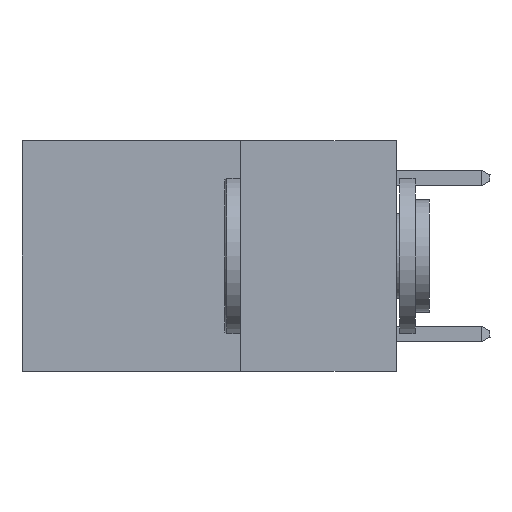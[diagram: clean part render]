
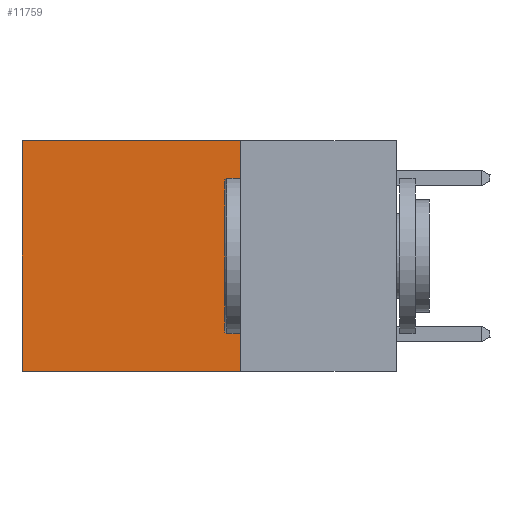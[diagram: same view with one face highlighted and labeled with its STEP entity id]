
A CAD part, left-side view. The second image highlights one B-rep face of the part: STEP entity #11759.
In plain terms, the highlighted planar face has unit normal (-1, 0, 0).
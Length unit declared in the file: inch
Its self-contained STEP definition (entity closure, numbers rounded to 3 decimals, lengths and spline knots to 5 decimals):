
#59 = DIRECTION ( 'NONE',  ( 0., 0., -1. ) ) ;
#110 = EDGE_CURVE ( 'NONE', #19671, #14846, #11611, .T. ) ;
#421 = DIRECTION ( 'NONE',  ( 0., 1., 0. ) ) ;
#1924 = DIRECTION ( 'NONE',  ( 0., 1., 0. ) ) ;
#2343 = CARTESIAN_POINT ( 'NONE',  ( 0.2625, 0.6, -0.37 ) ) ;
#3020 = CARTESIAN_POINT ( 'NONE',  ( 0.2625, 0.6, 0. ) ) ;
#3263 = LINE ( 'NONE', #19244, #4541 ) ;
#4438 = CARTESIAN_POINT ( 'NONE',  ( 0.2625, 0.25, 0. ) ) ;
#4541 = VECTOR ( 'NONE', #6297, 39.37008 ) ;
#6297 = DIRECTION ( 'NONE',  ( 0., 0., -1. ) ) ;
#6333 = CARTESIAN_POINT ( 'NONE',  ( 0.2625, 0.25, 0. ) ) ;
#6840 = VERTEX_POINT ( 'NONE', #6333 ) ;
#8144 = ORIENTED_EDGE ( 'NONE', *, *, #8543, .F. ) ;
#8543 = EDGE_CURVE ( 'NONE', #6840, #19671, #18642, .T. ) ;
#8999 = VECTOR ( 'NONE', #1924, 39.37008 ) ;
#9150 = AXIS2_PLACEMENT_3D ( 'NONE', #4438, #9249, #59 ) ;
#9249 = DIRECTION ( 'NONE',  ( 1., 0., 0. ) ) ;
#9448 = VERTEX_POINT ( 'NONE', #3020 ) ;
#9560 = PLANE ( 'NONE',  #9150 ) ;
#9979 = CARTESIAN_POINT ( 'NONE',  ( 0.2625, 0.25, 0. ) ) ;
#10255 = ORIENTED_EDGE ( 'NONE', *, *, #17837, .T. ) ;
#10469 = VECTOR ( 'NONE', #421, 39.37008 ) ;
#10628 = DIRECTION ( 'NONE',  ( 0., 0., -1. ) ) ;
#10818 = CARTESIAN_POINT ( 'NONE',  ( 0.2625, 0.25, 0. ) ) ;
#11611 = LINE ( 'NONE', #16772, #10469 ) ;
#11759 = ADVANCED_FACE ( 'NONE', ( #15549 ), #9560, .F. ) ;
#12289 = EDGE_LOOP ( 'NONE', ( #10255, #19639, #8144, #14338 ) ) ;
#13014 = LINE ( 'NONE', #9979, #8999 ) ;
#14338 = ORIENTED_EDGE ( 'NONE', *, *, #14637, .T. ) ;
#14637 = EDGE_CURVE ( 'NONE', #6840, #9448, #13014, .T. ) ;
#14846 = VERTEX_POINT ( 'NONE', #2343 ) ;
#15549 = FACE_OUTER_BOUND ( 'NONE', #12289, .T. ) ;
#16504 = VECTOR ( 'NONE', #10628, 39.37008 ) ;
#16772 = CARTESIAN_POINT ( 'NONE',  ( 0.2625, 0.25, -0.37 ) ) ;
#17837 = EDGE_CURVE ( 'NONE', #9448, #14846, #3263, .T. ) ;
#18642 = LINE ( 'NONE', #10818, #16504 ) ;
#19002 = CARTESIAN_POINT ( 'NONE',  ( 0.2625, 0.25, -0.37 ) ) ;
#19244 = CARTESIAN_POINT ( 'NONE',  ( 0.2625, 0.6, 0. ) ) ;
#19639 = ORIENTED_EDGE ( 'NONE', *, *, #110, .F. ) ;
#19671 = VERTEX_POINT ( 'NONE', #19002 ) ;
